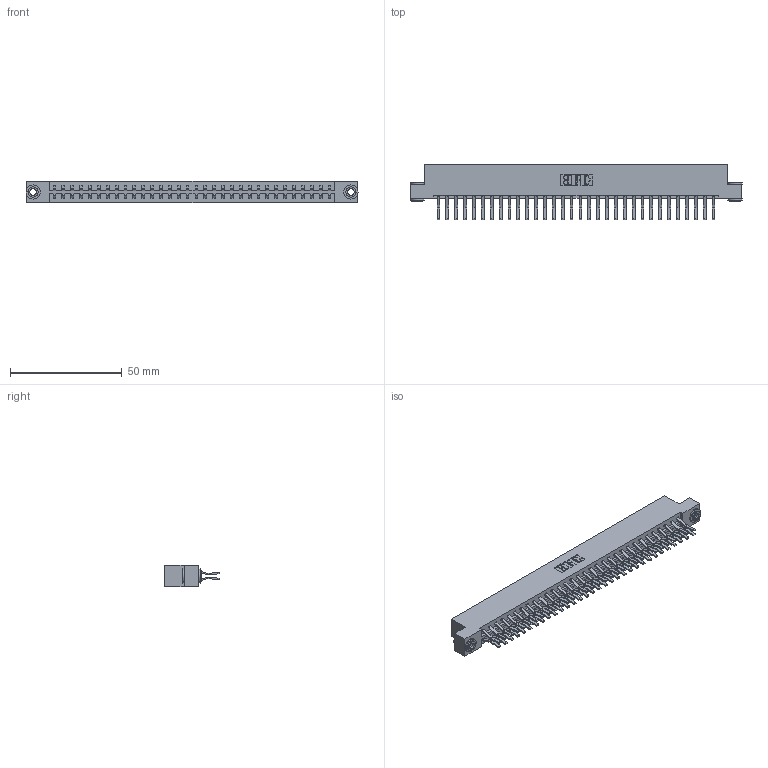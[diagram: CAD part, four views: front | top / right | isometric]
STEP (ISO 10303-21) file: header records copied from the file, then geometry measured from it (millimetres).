
FILE_DESCRIPTION (( 'STEP AP203' ), '1' );
FILE_NAME ('833-064-560-203.STEP', '2020-06-05T08:06:52', ( '' ), ( '' ), 'SwSTEP 2.0', 'SolidWorks 2020', '' );
FILE_SCHEMA (( 'CONFIG_CONTROL_DESIGN' ));
Length unit declared in the file: inch
Products named in the file (4): 345-250-002_345-250-002-102; 345-292-001_560 Tail; 833-064-560-203; 833 Part_Flush - .156 Dia - TH
Assembly tree (67 placements, depth 2):
  833-064-560-203
    833 Part_Flush - .156 Dia - TH
    345-292-001_560 Tail  x64
    345-250-002_345-250-002-102  x2
Bounding box: 148.34 x 24.78 x 9.4 mm (x, y, z)
Volume: 15489.6 mm3; surface area: 19622.7 mm2
Topology: 67 solids, 67 shells, 3608 faces, 10691 edges, 7038 vertices
Faces by surface type: plane 2384, cylinder 1216, cone 8
Entity records: 22618 total; most frequent: CARTESIAN_POINT 3737, ORIENTED_EDGE 3666, DIRECTION 3247, EDGE_CURVE 1833, LINE 1677, VECTOR 1677, VERTEX_POINT 1218, AXIS2_PLACEMENT_3D 785
